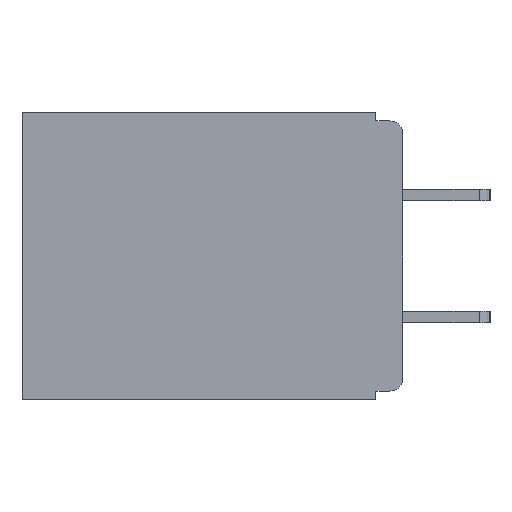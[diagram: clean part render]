
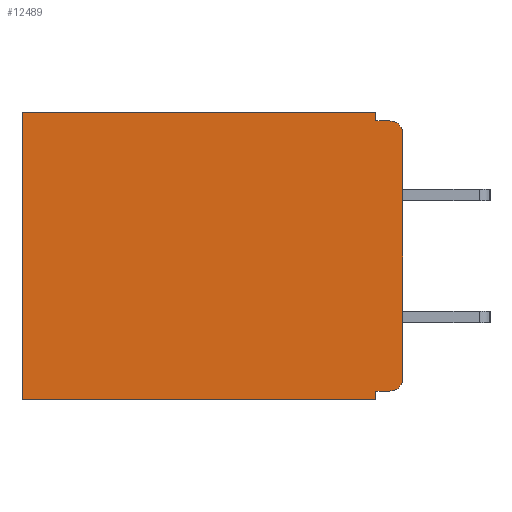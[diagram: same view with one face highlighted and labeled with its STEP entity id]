
A CAD part, left-side view. The second image highlights one B-rep face of the part: STEP entity #12489.
In plain terms, the highlighted planar face has unit normal (-1, 0, 0).
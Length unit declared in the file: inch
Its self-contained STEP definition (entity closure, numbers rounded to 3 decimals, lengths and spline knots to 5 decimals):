
#54 = AXIS2_PLACEMENT_3D ( 'NONE', #13174, #2529, #10062 ) ;
#322 = CARTESIAN_POINT ( 'NONE',  ( 0.3, 0.437, -0.33 ) ) ;
#369 = DIRECTION ( 'NONE',  ( 0., -1., 0. ) ) ;
#396 = DIRECTION ( 'NONE',  ( 0., 0., -1. ) ) ;
#592 = CARTESIAN_POINT ( 'NONE',  ( 0.3, 0.031, -0.33 ) ) ;
#994 = VERTEX_POINT ( 'NONE', #1264 ) ;
#1071 = CARTESIAN_POINT ( 'NONE',  ( 0.3, 0., -0.33 ) ) ;
#1085 = VERTEX_POINT ( 'NONE', #12790 ) ;
#1105 = DIRECTION ( 'NONE',  ( 0., 0., -1. ) ) ;
#1116 = VERTEX_POINT ( 'NONE', #10680 ) ;
#1127 = CARTESIAN_POINT ( 'NONE',  ( 0.3, 0.031, 0. ) ) ;
#1133 = VECTOR ( 'NONE', #369, 39.37008 ) ;
#1264 = CARTESIAN_POINT ( 'NONE',  ( 0.3, 0., -0.025 ) ) ;
#1374 = PLANE ( 'NONE',  #54 ) ;
#1387 = CARTESIAN_POINT ( 'NONE',  ( 0.3, 0.015, -0.01 ) ) ;
#1711 = VERTEX_POINT ( 'NONE', #4284 ) ;
#1879 = AXIS2_PLACEMENT_3D ( 'NONE', #12866, #6581, #13872 ) ;
#1926 = EDGE_CURVE ( 'NONE', #994, #6336, #6802, .T. ) ;
#2190 = EDGE_LOOP ( 'NONE', ( #4780, #7438, #7788, #5791, #6420, #6706, #13312, #5396, #5896, #8728 ) ) ;
#2286 = CARTESIAN_POINT ( 'NONE',  ( 0.3, 0., 0. ) ) ;
#2529 = DIRECTION ( 'NONE',  ( 1., 0., 0. ) ) ;
#3007 = LINE ( 'NONE', #1127, #11557 ) ;
#3100 = CARTESIAN_POINT ( 'NONE',  ( 0.3, 0.031, -0.32 ) ) ;
#3441 = VERTEX_POINT ( 'NONE', #7653 ) ;
#3784 = VECTOR ( 'NONE', #8029, 39.37008 ) ;
#3994 = CARTESIAN_POINT ( 'NONE',  ( 0.3, 0.015, -0.025 ) ) ;
#4141 = LINE ( 'NONE', #12598, #3784 ) ;
#4284 = CARTESIAN_POINT ( 'NONE',  ( 0.3, 0., -0.305 ) ) ;
#4421 = VERTEX_POINT ( 'NONE', #10346 ) ;
#4780 = ORIENTED_EDGE ( 'NONE', *, *, #6828, .F. ) ;
#4912 = EDGE_CURVE ( 'NONE', #8927, #10926, #4141, .T. ) ;
#5258 = VECTOR ( 'NONE', #396, 39.37008 ) ;
#5304 = VERTEX_POINT ( 'NONE', #7740 ) ;
#5314 = VECTOR ( 'NONE', #7699, 39.37008 ) ;
#5396 = ORIENTED_EDGE ( 'NONE', *, *, #12062, .F. ) ;
#5446 = DIRECTION ( 'NONE',  ( 0., 0., -1. ) ) ;
#5791 = ORIENTED_EDGE ( 'NONE', *, *, #8557, .F. ) ;
#5896 = ORIENTED_EDGE ( 'NONE', *, *, #4912, .F. ) ;
#6010 = CARTESIAN_POINT ( 'NONE',  ( 0.3, 0., -0.01 ) ) ;
#6024 = CIRCLE ( 'NONE', #1879, 0.015 ) ;
#6176 = DIRECTION ( 'NONE',  ( 0., 0., -1. ) ) ;
#6336 = VERTEX_POINT ( 'NONE', #1387 ) ;
#6420 = ORIENTED_EDGE ( 'NONE', *, *, #8689, .T. ) ;
#6581 = DIRECTION ( 'NONE',  ( -1., 0., 0. ) ) ;
#6706 = ORIENTED_EDGE ( 'NONE', *, *, #8583, .T. ) ;
#6802 = CIRCLE ( 'NONE', #12662, 0.015 ) ;
#6815 = DIRECTION ( 'NONE',  ( -1., 0., 0. ) ) ;
#6828 = EDGE_CURVE ( 'NONE', #994, #1711, #12903, .T. ) ;
#7141 = LINE ( 'NONE', #2286, #12379 ) ;
#7438 = ORIENTED_EDGE ( 'NONE', *, *, #1926, .T. ) ;
#7653 = CARTESIAN_POINT ( 'NONE',  ( 0.3, 0.031, 0. ) ) ;
#7699 = DIRECTION ( 'NONE',  ( 0., 1., 0. ) ) ;
#7740 = CARTESIAN_POINT ( 'NONE',  ( 0.3, 0.031, -0.33 ) ) ;
#7788 = ORIENTED_EDGE ( 'NONE', *, *, #11309, .F. ) ;
#8029 = DIRECTION ( 'NONE',  ( 0., 1., 0. ) ) ;
#8326 = FACE_OUTER_BOUND ( 'NONE', #2190, .T. ) ;
#8557 = EDGE_CURVE ( 'NONE', #3441, #1085, #3007, .T. ) ;
#8583 = EDGE_CURVE ( 'NONE', #4421, #1116, #13643, .T. ) ;
#8689 = EDGE_CURVE ( 'NONE', #3441, #4421, #7141, .T. ) ;
#8728 = ORIENTED_EDGE ( 'NONE', *, *, #12282, .T. ) ;
#8927 = VERTEX_POINT ( 'NONE', #11353 ) ;
#8974 = LINE ( 'NONE', #592, #11125 ) ;
#9012 = CARTESIAN_POINT ( 'NONE',  ( 0.3, 0., -0.33 ) ) ;
#9814 = DIRECTION ( 'NONE',  ( 0., 1., 0. ) ) ;
#10062 = DIRECTION ( 'NONE',  ( 0., 0., -1. ) ) ;
#10346 = CARTESIAN_POINT ( 'NONE',  ( 0.3, 0.437, 0. ) ) ;
#10680 = CARTESIAN_POINT ( 'NONE',  ( 0.3, 0.437, -0.33 ) ) ;
#10926 = VERTEX_POINT ( 'NONE', #3100 ) ;
#11125 = VECTOR ( 'NONE', #6176, 39.37008 ) ;
#11309 = EDGE_CURVE ( 'NONE', #1085, #6336, #12624, .T. ) ;
#11353 = CARTESIAN_POINT ( 'NONE',  ( 0.3, 0.015, -0.32 ) ) ;
#11445 = DIRECTION ( 'NONE',  ( 0., 0., -1. ) ) ;
#11557 = VECTOR ( 'NONE', #1105, 39.37008 ) ;
#12062 = EDGE_CURVE ( 'NONE', #10926, #5304, #8974, .T. ) ;
#12282 = EDGE_CURVE ( 'NONE', #8927, #1711, #6024, .T. ) ;
#12332 = EDGE_CURVE ( 'NONE', #5304, #1116, #13387, .T. ) ;
#12379 = VECTOR ( 'NONE', #9814, 39.37008 ) ;
#12489 = ADVANCED_FACE ( 'NONE', ( #8326 ), #1374, .F. ) ;
#12586 = VECTOR ( 'NONE', #11445, 39.37008 ) ;
#12598 = CARTESIAN_POINT ( 'NONE',  ( 0.3, 0., -0.32 ) ) ;
#12624 = LINE ( 'NONE', #6010, #1133 ) ;
#12662 = AXIS2_PLACEMENT_3D ( 'NONE', #3994, #6815, #5446 ) ;
#12790 = CARTESIAN_POINT ( 'NONE',  ( 0.3, 0.031, -0.01 ) ) ;
#12866 = CARTESIAN_POINT ( 'NONE',  ( 0.3, 0.015, -0.305 ) ) ;
#12903 = LINE ( 'NONE', #9012, #12586 ) ;
#13174 = CARTESIAN_POINT ( 'NONE',  ( 0.3, 0., -0.33 ) ) ;
#13312 = ORIENTED_EDGE ( 'NONE', *, *, #12332, .F. ) ;
#13387 = LINE ( 'NONE', #1071, #5314 ) ;
#13643 = LINE ( 'NONE', #322, #5258 ) ;
#13872 = DIRECTION ( 'NONE',  ( 0., 0., -1. ) ) ;
